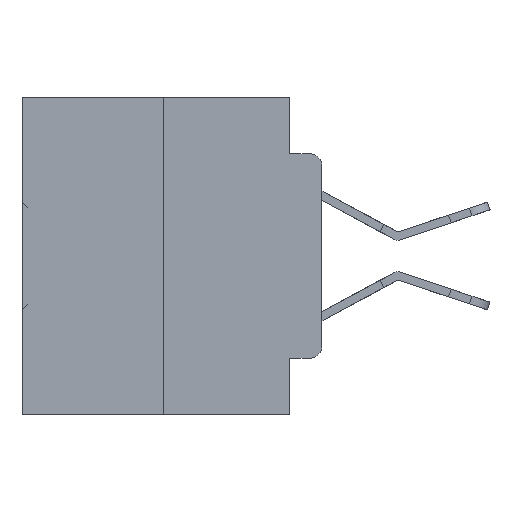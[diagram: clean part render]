
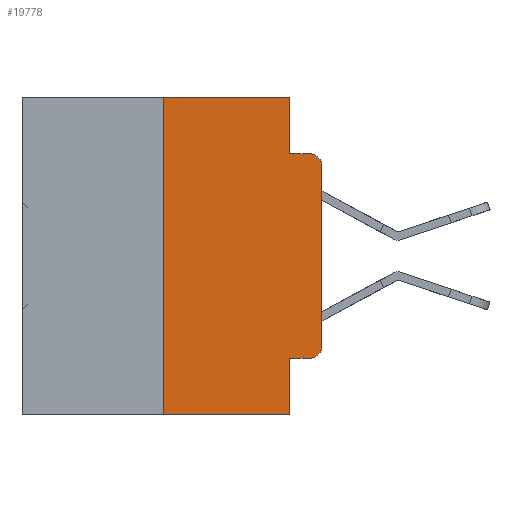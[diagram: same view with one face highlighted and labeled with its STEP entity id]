
A CAD part, left-side view. The second image highlights one B-rep face of the part: STEP entity #19778.
In plain terms, the highlighted planar face has unit normal (-1, 0, 0).
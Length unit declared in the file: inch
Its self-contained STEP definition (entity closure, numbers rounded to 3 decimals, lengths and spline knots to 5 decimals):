
#52 = DIRECTION ( 'NONE',  ( 0., 0., -1. ) ) ;
#195 = VERTEX_POINT ( 'NONE', #10426 ) ;
#533 = CARTESIAN_POINT ( 'NONE',  ( 0., 0.051, 0. ) ) ;
#1094 = EDGE_LOOP ( 'NONE', ( #1156, #26716, #34481, #28083, #28991, #24965, #29856, #23109, #2150, #11950 ) ) ;
#1156 = ORIENTED_EDGE ( 'NONE', *, *, #34047, .T. ) ;
#1648 = VECTOR ( 'NONE', #19621, 39.37008 ) ;
#2150 = ORIENTED_EDGE ( 'NONE', *, *, #34757, .T. ) ;
#2201 = DIRECTION ( 'NONE',  ( 0., -1., 0. ) ) ;
#2401 = EDGE_CURVE ( 'NONE', #11046, #13353, #13526, .T. ) ;
#3154 = CIRCLE ( 'NONE', #28438, 0.02 ) ;
#3197 = CARTESIAN_POINT ( 'NONE',  ( 0., 0.051, -0.0885 ) ) ;
#3206 = CARTESIAN_POINT ( 'NONE',  ( 0., 0., -0.1085 ) ) ;
#3360 = VERTEX_POINT ( 'NONE', #20109 ) ;
#4405 = VECTOR ( 'NONE', #13006, 39.37008 ) ;
#5641 = VECTOR ( 'NONE', #26512, 39.37008 ) ;
#6705 = VERTEX_POINT ( 'NONE', #10933 ) ;
#7380 = CARTESIAN_POINT ( 'NONE',  ( 0., 0.051, -0.4115 ) ) ;
#7604 = VERTEX_POINT ( 'NONE', #3206 ) ;
#9320 = FACE_OUTER_BOUND ( 'NONE', #1094, .T. ) ;
#9642 = VECTOR ( 'NONE', #33769, 39.37008 ) ;
#10414 = EDGE_CURVE ( 'NONE', #3360, #6705, #33058, .T. ) ;
#10426 = CARTESIAN_POINT ( 'NONE',  ( 0., 0., -0.3915 ) ) ;
#10933 = CARTESIAN_POINT ( 'NONE',  ( 0., 0.25, 0. ) ) ;
#11046 = VERTEX_POINT ( 'NONE', #7380 ) ;
#11950 = ORIENTED_EDGE ( 'NONE', *, *, #23092, .T. ) ;
#12266 = LINE ( 'NONE', #24778, #4405 ) ;
#12438 = CARTESIAN_POINT ( 'NONE',  ( 0., 0.02, -0.0885 ) ) ;
#12771 = CARTESIAN_POINT ( 'NONE',  ( 0., 0.473, 0. ) ) ;
#12851 = LINE ( 'NONE', #19736, #20804 ) ;
#12894 = DIRECTION ( 'NONE',  ( 0., 0., -1. ) ) ;
#13006 = DIRECTION ( 'NONE',  ( 0., -1., 0. ) ) ;
#13110 = DIRECTION ( 'NONE',  ( 0., -1., 0. ) ) ;
#13353 = VERTEX_POINT ( 'NONE', #37951 ) ;
#13526 = LINE ( 'NONE', #533, #5641 ) ;
#14464 = DIRECTION ( 'NONE',  ( -1., 0., 0. ) ) ;
#14480 = EDGE_CURVE ( 'NONE', #3360, #13353, #25490, .T. ) ;
#16125 = VERTEX_POINT ( 'NONE', #3197 ) ;
#16444 = EDGE_CURVE ( 'NONE', #35171, #16125, #25363, .T. ) ;
#16631 = CARTESIAN_POINT ( 'NONE',  ( 0., 0.051, 0. ) ) ;
#17408 = VERTEX_POINT ( 'NONE', #35417 ) ;
#18150 = DIRECTION ( 'NONE',  ( -1., 0., 0. ) ) ;
#18603 = DIRECTION ( 'NONE',  ( 0., 0., 1. ) ) ;
#18617 = VECTOR ( 'NONE', #13110, 39.37008 ) ;
#19433 = AXIS2_PLACEMENT_3D ( 'NONE', #31977, #14464, #34924 ) ;
#19621 = DIRECTION ( 'NONE',  ( 0., 0., -1. ) ) ;
#19736 = CARTESIAN_POINT ( 'NONE',  ( 0., 0.473, 0. ) ) ;
#19778 = ADVANCED_FACE ( 'NONE', ( #9320 ), #21778, .F. ) ;
#20109 = CARTESIAN_POINT ( 'NONE',  ( 0., 0.25, -0.5 ) ) ;
#20421 = EDGE_CURVE ( 'NONE', #16125, #24539, #27212, .T. ) ;
#20804 = VECTOR ( 'NONE', #22677, 39.37008 ) ;
#21778 = PLANE ( 'NONE',  #22297 ) ;
#22297 = AXIS2_PLACEMENT_3D ( 'NONE', #12771, #30465, #12894 ) ;
#22677 = DIRECTION ( 'NONE',  ( 0., -1., 0. ) ) ;
#23028 = CARTESIAN_POINT ( 'NONE',  ( 0., 0.473, -0.5 ) ) ;
#23092 = EDGE_CURVE ( 'NONE', #17408, #195, #29717, .T. ) ;
#23109 = ORIENTED_EDGE ( 'NONE', *, *, #2401, .F. ) ;
#24539 = VERTEX_POINT ( 'NONE', #12438 ) ;
#24610 = VECTOR ( 'NONE', #2201, 39.37008 ) ;
#24778 = CARTESIAN_POINT ( 'NONE',  ( 0., 0.051, -0.4115 ) ) ;
#24874 = CARTESIAN_POINT ( 'NONE',  ( 0., 0.051, -0.0885 ) ) ;
#24965 = ORIENTED_EDGE ( 'NONE', *, *, #10414, .F. ) ;
#25363 = LINE ( 'NONE', #16631, #1648 ) ;
#25490 = LINE ( 'NONE', #23028, #24610 ) ;
#26220 = EDGE_CURVE ( 'NONE', #7604, #24539, #3154, .T. ) ;
#26512 = DIRECTION ( 'NONE',  ( 0., 0., -1. ) ) ;
#26716 = ORIENTED_EDGE ( 'NONE', *, *, #26220, .T. ) ;
#27043 = EDGE_CURVE ( 'NONE', #6705, #35171, #12851, .T. ) ;
#27212 = LINE ( 'NONE', #24874, #18617 ) ;
#27875 = CARTESIAN_POINT ( 'NONE',  ( 0., 0.25, 0. ) ) ;
#28083 = ORIENTED_EDGE ( 'NONE', *, *, #16444, .F. ) ;
#28438 = AXIS2_PLACEMENT_3D ( 'NONE', #35540, #18150, #52 ) ;
#28991 = ORIENTED_EDGE ( 'NONE', *, *, #27043, .F. ) ;
#29258 = CARTESIAN_POINT ( 'NONE',  ( 0., 0.051, 0. ) ) ;
#29717 = CIRCLE ( 'NONE', #19433, 0.02 ) ;
#29856 = ORIENTED_EDGE ( 'NONE', *, *, #14480, .T. ) ;
#30465 = DIRECTION ( 'NONE',  ( 1., 0., 0. ) ) ;
#31977 = CARTESIAN_POINT ( 'NONE',  ( 0., 0.02, -0.3915 ) ) ;
#32090 = LINE ( 'NONE', #35879, #38022 ) ;
#33058 = LINE ( 'NONE', #27875, #9642 ) ;
#33769 = DIRECTION ( 'NONE',  ( 0., 0., 1. ) ) ;
#34047 = EDGE_CURVE ( 'NONE', #195, #7604, #32090, .T. ) ;
#34481 = ORIENTED_EDGE ( 'NONE', *, *, #20421, .F. ) ;
#34757 = EDGE_CURVE ( 'NONE', #11046, #17408, #12266, .T. ) ;
#34924 = DIRECTION ( 'NONE',  ( 0., 0., -1. ) ) ;
#35171 = VERTEX_POINT ( 'NONE', #29258 ) ;
#35417 = CARTESIAN_POINT ( 'NONE',  ( 0., 0.02, -0.4115 ) ) ;
#35540 = CARTESIAN_POINT ( 'NONE',  ( 0., 0.02, -0.1085 ) ) ;
#35879 = CARTESIAN_POINT ( 'NONE',  ( 0., 0., 0. ) ) ;
#37951 = CARTESIAN_POINT ( 'NONE',  ( 0., 0.051, -0.5 ) ) ;
#38022 = VECTOR ( 'NONE', #18603, 39.37008 ) ;
